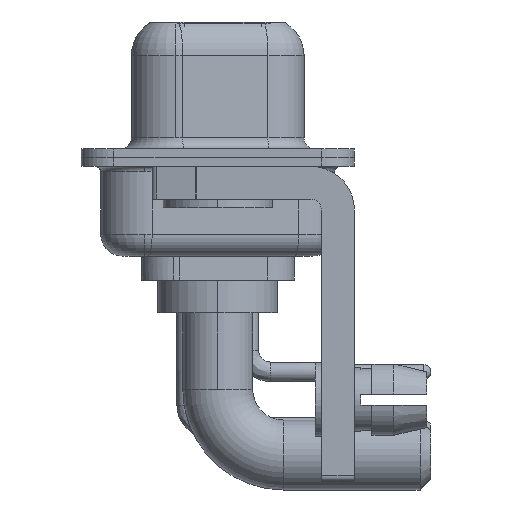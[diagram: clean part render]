
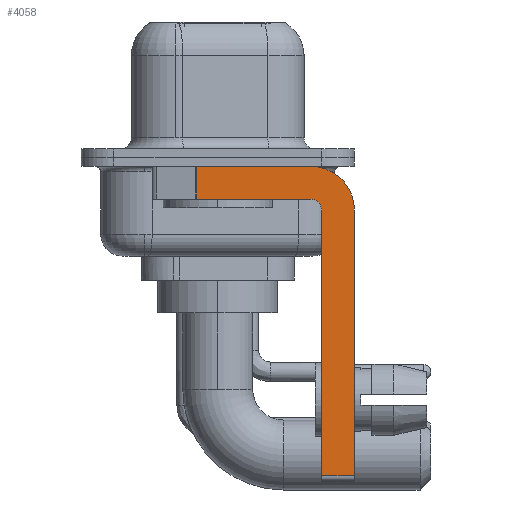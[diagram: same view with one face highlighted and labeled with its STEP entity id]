
A CAD part, left-side view. The second image highlights one B-rep face of the part: STEP entity #4058.
In plain terms, the highlighted planar face has unit normal (-1, 0, 0).
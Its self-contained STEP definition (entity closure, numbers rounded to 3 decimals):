
#425 = CARTESIAN_POINT ( 'NONE',  ( -2.9, 3., -0.4 ) ) ;
#964 = VERTEX_POINT ( 'NONE', #8001 ) ;
#1062 = EDGE_CURVE ( 'NONE', #13619, #19147, #18498, .T. ) ;
#1400 = DIRECTION ( 'NONE',  ( 0., 1., 0. ) ) ;
#1731 = LINE ( 'NONE', #6404, #2529 ) ;
#2214 = CIRCLE ( 'NONE', #9721, 2. ) ;
#2354 = ORIENTED_EDGE ( 'NONE', *, *, #11647, .F. ) ;
#2529 = VECTOR ( 'NONE', #6605, 1000. ) ;
#2668 = VERTEX_POINT ( 'NONE', #4284 ) ;
#2883 = LINE ( 'NONE', #18171, #10238 ) ;
#3734 = CARTESIAN_POINT ( 'NONE',  ( -2.9, -4.25, -14.55 ) ) ;
#3802 = VECTOR ( 'NONE', #13942, 1000. ) ;
#3993 = CARTESIAN_POINT ( 'NONE',  ( -2.9, 0.978, -0.4 ) ) ;
#4058 = ADVANCED_FACE ( 'NONE', ( #17980 ), #16584, .F. ) ;
#4284 = CARTESIAN_POINT ( 'NONE',  ( -2.9, -4.75, -2.4 ) ) ;
#4385 = CARTESIAN_POINT ( 'NONE',  ( -2.9, -4.25, -2.4 ) ) ;
#4416 = VERTEX_POINT ( 'NONE', #7548 ) ;
#5087 = DIRECTION ( 'NONE',  ( -1., 0., 0. ) ) ;
#5190 = CARTESIAN_POINT ( 'NONE',  ( -2.9, -6.25, -14.55 ) ) ;
#5215 = DIRECTION ( 'NONE',  ( 0., 0., 1. ) ) ;
#5547 = VECTOR ( 'NONE', #18159, 1000. ) ;
#5621 = EDGE_CURVE ( 'NONE', #2668, #11792, #15969, .T. ) ;
#6404 = CARTESIAN_POINT ( 'NONE',  ( -2.9, 0.978, -1.9 ) ) ;
#6549 = EDGE_CURVE ( 'NONE', #4416, #2668, #12871, .T. ) ;
#6605 = DIRECTION ( 'NONE',  ( 0., 0., -1. ) ) ;
#6963 = CARTESIAN_POINT ( 'NONE',  ( -2.9, -6.25, -2.4 ) ) ;
#7048 = EDGE_LOOP ( 'NONE', ( #7353, #10658, #9211, #12109, #11623, #13187, #17200, #2354 ) ) ;
#7121 = VERTEX_POINT ( 'NONE', #5190 ) ;
#7353 = ORIENTED_EDGE ( 'NONE', *, *, #1062, .F. ) ;
#7548 = CARTESIAN_POINT ( 'NONE',  ( -2.9, -4.75, -14.55 ) ) ;
#8001 = CARTESIAN_POINT ( 'NONE',  ( -2.9, -6.25, -2.4 ) ) ;
#9211 = ORIENTED_EDGE ( 'NONE', *, *, #15211, .F. ) ;
#9721 = AXIS2_PLACEMENT_3D ( 'NONE', #11002, #15630, #10799 ) ;
#10238 = VECTOR ( 'NONE', #1400, 1000. ) ;
#10324 = VERTEX_POINT ( 'NONE', #14515 ) ;
#10658 = ORIENTED_EDGE ( 'NONE', *, *, #11696, .T. ) ;
#10799 = DIRECTION ( 'NONE',  ( 0., 0., -1. ) ) ;
#11002 = CARTESIAN_POINT ( 'NONE',  ( -2.9, -4.25, -2.4 ) ) ;
#11063 = EDGE_CURVE ( 'NONE', #4416, #7121, #13181, .T. ) ;
#11237 = AXIS2_PLACEMENT_3D ( 'NONE', #17290, #5087, #15900 ) ;
#11623 = ORIENTED_EDGE ( 'NONE', *, *, #6549, .F. ) ;
#11647 = EDGE_CURVE ( 'NONE', #19147, #964, #2214, .T. ) ;
#11696 = EDGE_CURVE ( 'NONE', #13619, #10324, #1731, .T. ) ;
#11792 = VERTEX_POINT ( 'NONE', #12962 ) ;
#12089 = VECTOR ( 'NONE', #18830, 1000. ) ;
#12109 = ORIENTED_EDGE ( 'NONE', *, *, #5621, .F. ) ;
#12871 = LINE ( 'NONE', #17705, #15681 ) ;
#12962 = CARTESIAN_POINT ( 'NONE',  ( -2.9, -4.25, -1.9 ) ) ;
#13181 = LINE ( 'NONE', #3734, #12089 ) ;
#13187 = ORIENTED_EDGE ( 'NONE', *, *, #11063, .T. ) ;
#13388 = AXIS2_PLACEMENT_3D ( 'NONE', #4385, #18065, #18169 ) ;
#13619 = VERTEX_POINT ( 'NONE', #3993 ) ;
#13942 = DIRECTION ( 'NONE',  ( 0., -1., 0. ) ) ;
#14515 = CARTESIAN_POINT ( 'NONE',  ( -2.9, 0.978, -1.9 ) ) ;
#15211 = EDGE_CURVE ( 'NONE', #11792, #10324, #2883, .T. ) ;
#15630 = DIRECTION ( 'NONE',  ( 1., 0., 0. ) ) ;
#15681 = VECTOR ( 'NONE', #5215, 1000. ) ;
#15900 = DIRECTION ( 'NONE',  ( 0., 0., 1. ) ) ;
#15969 = CIRCLE ( 'NONE', #11237, 0.5 ) ;
#16584 = PLANE ( 'NONE',  #13388 ) ;
#17200 = ORIENTED_EDGE ( 'NONE', *, *, #18063, .F. ) ;
#17290 = CARTESIAN_POINT ( 'NONE',  ( -2.9, -4.25, -2.4 ) ) ;
#17293 = CARTESIAN_POINT ( 'NONE',  ( -2.9, -4.25, -0.4 ) ) ;
#17705 = CARTESIAN_POINT ( 'NONE',  ( -2.9, -4.75, -14.8 ) ) ;
#17980 = FACE_OUTER_BOUND ( 'NONE', #7048, .T. ) ;
#18063 = EDGE_CURVE ( 'NONE', #964, #7121, #19467, .T. ) ;
#18065 = DIRECTION ( 'NONE',  ( 1., 0., 0. ) ) ;
#18159 = DIRECTION ( 'NONE',  ( 0., 0., -1. ) ) ;
#18169 = DIRECTION ( 'NONE',  ( 0., 0., -1. ) ) ;
#18171 = CARTESIAN_POINT ( 'NONE',  ( -2.9, -4.25, -1.9 ) ) ;
#18498 = LINE ( 'NONE', #425, #3802 ) ;
#18830 = DIRECTION ( 'NONE',  ( 0., -1., 0. ) ) ;
#19147 = VERTEX_POINT ( 'NONE', #17293 ) ;
#19467 = LINE ( 'NONE', #6963, #5547 ) ;
